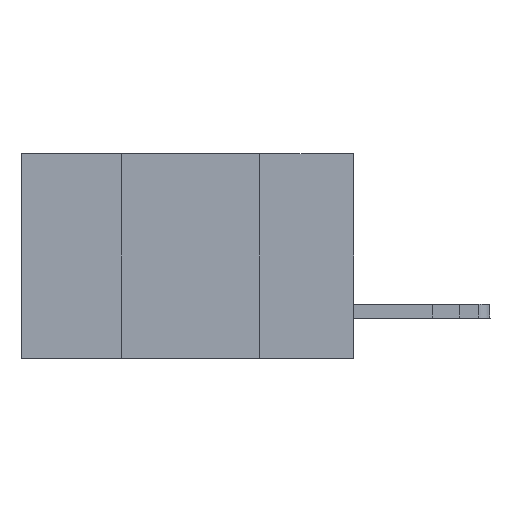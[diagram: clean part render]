
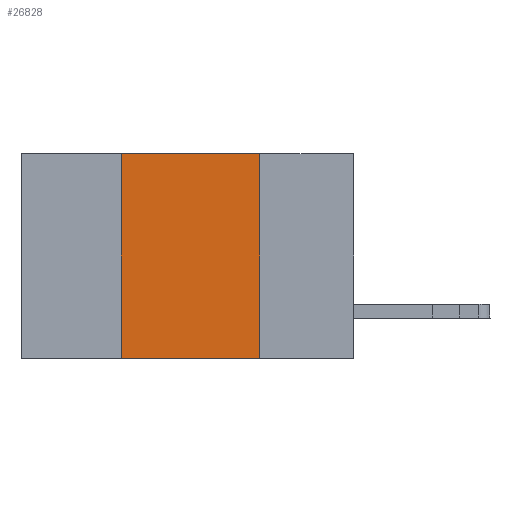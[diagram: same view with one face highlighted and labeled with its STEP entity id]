
A CAD part, left-side view. The second image highlights one B-rep face of the part: STEP entity #26828.
In plain terms, the highlighted planar face has unit normal (-1, 0, 0).
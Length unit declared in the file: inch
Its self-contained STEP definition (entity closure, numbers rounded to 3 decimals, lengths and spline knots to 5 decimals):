
#153 = VERTEX_POINT ( 'NONE', #18245 ) ;
#565 = VECTOR ( 'NONE', #14593, 39.37008 ) ;
#1780 = EDGE_CURVE ( 'NONE', #153, #28418, #24781, .T. ) ;
#1828 = ORIENTED_EDGE ( 'NONE', *, *, #19935, .F. ) ;
#2965 = LINE ( 'NONE', #22655, #15095 ) ;
#3247 = DIRECTION ( 'NONE',  ( 0., -1., 0. ) ) ;
#3355 = CARTESIAN_POINT ( 'NONE',  ( 0., 0.6, 0. ) ) ;
#3407 = DIRECTION ( 'NONE',  ( 0., 0., -1. ) ) ;
#3738 = DIRECTION ( 'NONE',  ( 1., 0., 0. ) ) ;
#4847 = CARTESIAN_POINT ( 'NONE',  ( 0., 0.6, -0.37 ) ) ;
#4894 = VECTOR ( 'NONE', #26432, 39.37008 ) ;
#5995 = VECTOR ( 'NONE', #3247, 39.37008 ) ;
#7334 = VERTEX_POINT ( 'NONE', #19159 ) ;
#9996 = VERTEX_POINT ( 'NONE', #29080 ) ;
#10496 = ORIENTED_EDGE ( 'NONE', *, *, #1780, .T. ) ;
#13196 = LINE ( 'NONE', #3355, #5995 ) ;
#13456 = LINE ( 'NONE', #14499, #565 ) ;
#14113 = EDGE_CURVE ( 'NONE', #7334, #9996, #13196, .T. ) ;
#14499 = CARTESIAN_POINT ( 'NONE',  ( 0., 0.42, 0. ) ) ;
#14593 = DIRECTION ( 'NONE',  ( 0., 0., 1. ) ) ;
#15095 = VECTOR ( 'NONE', #3407, 39.37008 ) ;
#15675 = ORIENTED_EDGE ( 'NONE', *, *, #25952, .F. ) ;
#18131 = CARTESIAN_POINT ( 'NONE',  ( 0., 0.6, 0. ) ) ;
#18245 = CARTESIAN_POINT ( 'NONE',  ( 0., 0.42, -0.37 ) ) ;
#19159 = CARTESIAN_POINT ( 'NONE',  ( 0., 0.42, 0. ) ) ;
#19935 = EDGE_CURVE ( 'NONE', #9996, #28418, #2965, .T. ) ;
#20482 = EDGE_LOOP ( 'NONE', ( #1828, #30722, #15675, #10496 ) ) ;
#20535 = DIRECTION ( 'NONE',  ( 0., 0., -1. ) ) ;
#22186 = CARTESIAN_POINT ( 'NONE',  ( 0., 0.17, -0.37 ) ) ;
#22655 = CARTESIAN_POINT ( 'NONE',  ( 0., 0.17, 0. ) ) ;
#24254 = AXIS2_PLACEMENT_3D ( 'NONE', #18131, #3738, #20535 ) ;
#24781 = LINE ( 'NONE', #4847, #4894 ) ;
#25282 = PLANE ( 'NONE',  #24254 ) ;
#25952 = EDGE_CURVE ( 'NONE', #153, #7334, #13456, .T. ) ;
#26432 = DIRECTION ( 'NONE',  ( 0., -1., 0. ) ) ;
#26828 = ADVANCED_FACE ( 'NONE', ( #30863 ), #25282, .F. ) ;
#28418 = VERTEX_POINT ( 'NONE', #22186 ) ;
#29080 = CARTESIAN_POINT ( 'NONE',  ( 0., 0.17, 0. ) ) ;
#30722 = ORIENTED_EDGE ( 'NONE', *, *, #14113, .F. ) ;
#30863 = FACE_OUTER_BOUND ( 'NONE', #20482, .T. ) ;
